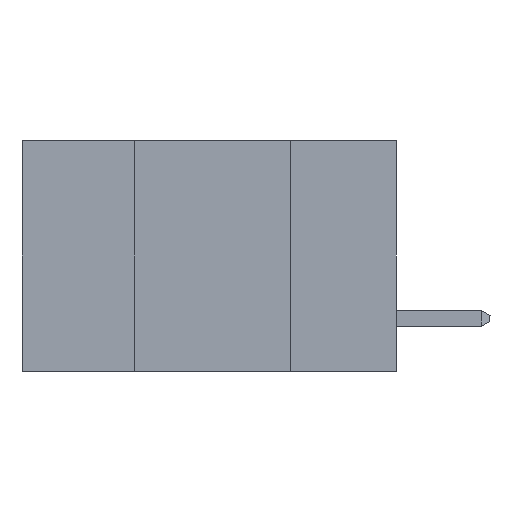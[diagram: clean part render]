
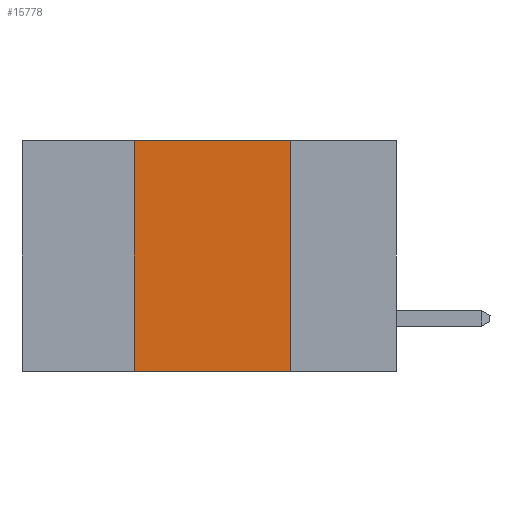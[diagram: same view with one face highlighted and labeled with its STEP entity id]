
A CAD part, left-side view. The second image highlights one B-rep face of the part: STEP entity #15778.
In plain terms, the highlighted planar face has unit normal (-1, 0, 0).
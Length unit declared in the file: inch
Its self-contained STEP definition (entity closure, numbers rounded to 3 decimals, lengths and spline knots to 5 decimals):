
#3108 = CARTESIAN_POINT ( 'NONE',  ( 0., 0.42, 0. ) ) ;
#3333 = ORIENTED_EDGE ( 'NONE', *, *, #8394, .F. ) ;
#3496 = EDGE_CURVE ( 'NONE', #14321, #7361, #18278, .T. ) ;
#4913 = DIRECTION ( 'NONE',  ( 0., -1., 0. ) ) ;
#5076 = CARTESIAN_POINT ( 'NONE',  ( 0., 0.6, -0.37 ) ) ;
#5402 = VERTEX_POINT ( 'NONE', #13667 ) ;
#5622 = VERTEX_POINT ( 'NONE', #3108 ) ;
#6531 = DIRECTION ( 'NONE',  ( 0., 0., -1. ) ) ;
#6580 = CARTESIAN_POINT ( 'NONE',  ( 0., 0.17, -0.37 ) ) ;
#7361 = VERTEX_POINT ( 'NONE', #12502 ) ;
#8394 = EDGE_CURVE ( 'NONE', #5402, #5622, #21091, .T. ) ;
#8400 = VECTOR ( 'NONE', #8954, 39.37008 ) ;
#8770 = VECTOR ( 'NONE', #6531, 39.37008 ) ;
#8951 = DIRECTION ( 'NONE',  ( 1., 0., 0. ) ) ;
#8954 = DIRECTION ( 'NONE',  ( 0., -1., 0. ) ) ;
#9096 = CARTESIAN_POINT ( 'NONE',  ( 0., 0.6, 0. ) ) ;
#9598 = EDGE_CURVE ( 'NONE', #5402, #7361, #18008, .T. ) ;
#10008 = CARTESIAN_POINT ( 'NONE',  ( 0., 0.17, 0. ) ) ;
#11082 = VECTOR ( 'NONE', #18939, 39.37008 ) ;
#11848 = ORIENTED_EDGE ( 'NONE', *, *, #12457, .F. ) ;
#12457 = EDGE_CURVE ( 'NONE', #5622, #14321, #22479, .T. ) ;
#12502 = CARTESIAN_POINT ( 'NONE',  ( 0., 0.17, -0.37 ) ) ;
#13667 = CARTESIAN_POINT ( 'NONE',  ( 0., 0.42, -0.37 ) ) ;
#14321 = VERTEX_POINT ( 'NONE', #10008 ) ;
#14687 = AXIS2_PLACEMENT_3D ( 'NONE', #17839, #8951, #21354 ) ;
#15778 = ADVANCED_FACE ( 'NONE', ( #21408 ), #19624, .F. ) ;
#17689 = ORIENTED_EDGE ( 'NONE', *, *, #9598, .T. ) ;
#17839 = CARTESIAN_POINT ( 'NONE',  ( 0., 0.6, 0. ) ) ;
#18008 = LINE ( 'NONE', #5076, #20484 ) ;
#18278 = LINE ( 'NONE', #6580, #8770 ) ;
#18939 = DIRECTION ( 'NONE',  ( 0., 0., 1. ) ) ;
#19624 = PLANE ( 'NONE',  #14687 ) ;
#20484 = VECTOR ( 'NONE', #4913, 39.37008 ) ;
#20708 = EDGE_LOOP ( 'NONE', ( #21275, #11848, #3333, #17689 ) ) ;
#20904 = CARTESIAN_POINT ( 'NONE',  ( 0., 0.42, -0.37 ) ) ;
#21091 = LINE ( 'NONE', #20904, #11082 ) ;
#21275 = ORIENTED_EDGE ( 'NONE', *, *, #3496, .F. ) ;
#21354 = DIRECTION ( 'NONE',  ( 0., 0., -1. ) ) ;
#21408 = FACE_OUTER_BOUND ( 'NONE', #20708, .T. ) ;
#22479 = LINE ( 'NONE', #9096, #8400 ) ;
